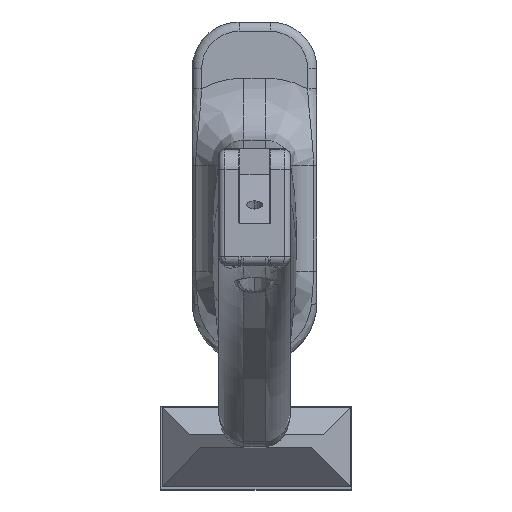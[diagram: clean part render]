
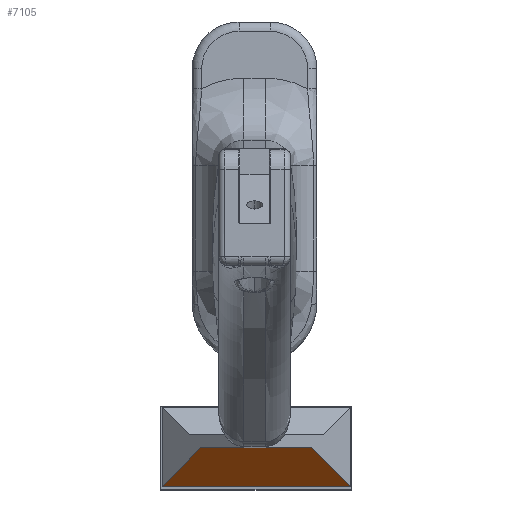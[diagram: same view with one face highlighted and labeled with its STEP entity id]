
A CAD part, top view. The second image highlights one B-rep face of the part: STEP entity #7105.
In plain terms, the highlighted planar face has unit normal (0, -0.707, 0.707).
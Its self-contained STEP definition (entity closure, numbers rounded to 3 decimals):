
#2498=DIRECTION('',(0.577,0.577,0.577));
#2499=VECTOR('',#2498,21.651);
#2500=CARTESIAN_POINT('',(-29.709,-101.607,
-227.026));
#2501=LINE('',#2500,#2499);
#2506=DIRECTION('',(-1.,0.,0.));
#2507=VECTOR('',#2506,35.519);
#2508=CARTESIAN_POINT('',(18.309,-89.107,
-214.526));
#2509=LINE('',#2508,#2507);
#2518=DIRECTION('',(-0.577,0.577,0.577));
#2519=VECTOR('',#2518,21.651);
#2520=CARTESIAN_POINT('',(30.809,-101.607,
-227.026));
#2521=LINE('',#2520,#2519);
#2684=DIRECTION('',(-1.,0.,0.));
#2685=VECTOR('',#2684,60.519);
#2686=CARTESIAN_POINT('',(30.809,-101.607,
-227.026));
#2687=LINE('',#2686,#2685);
#3098=CARTESIAN_POINT('',(30.809,-101.607,
-227.026));
#3099=CARTESIAN_POINT('',(-29.709,-101.607,
-227.026));
#3100=VERTEX_POINT('',#3098);
#3101=VERTEX_POINT('',#3099);
#3116=CARTESIAN_POINT('',(18.309,-89.107,
-214.526));
#3117=VERTEX_POINT('',#3116);
#3118=CARTESIAN_POINT('',(-17.209,-89.107,
-214.526));
#3119=VERTEX_POINT('',#3118);
#7092=CARTESIAN_POINT('',(0.,-95.357,
-220.776));
#7093=DIRECTION('',(0.,-0.707,0.707));
#7094=DIRECTION('',(0.,0.707,0.707));
#7095=AXIS2_PLACEMENT_3D('',#7092,#7093,#7094);
#7096=PLANE('',#7095);
#7097=ORIENTED_EDGE('',*,*,#7079,.F.);
#7099=ORIENTED_EDGE('',*,*,#7098,.F.);
#7101=ORIENTED_EDGE('',*,*,#7100,.T.);
#7102=ORIENTED_EDGE('',*,*,#7064,.T.);
#7103=EDGE_LOOP('',(#7097,#7099,#7101,#7102));
#7104=FACE_OUTER_BOUND('',#7103,.F.);
#7105=ADVANCED_FACE('',(#7104),#7096,.T.);
#7064=EDGE_CURVE('',#3101,#3119,#2501,.T.);
#7079=EDGE_CURVE('',#3117,#3119,#2509,.T.);
#7098=EDGE_CURVE('',#3100,#3117,#2521,.T.);
#7100=EDGE_CURVE('',#3100,#3101,#2687,.T.);
